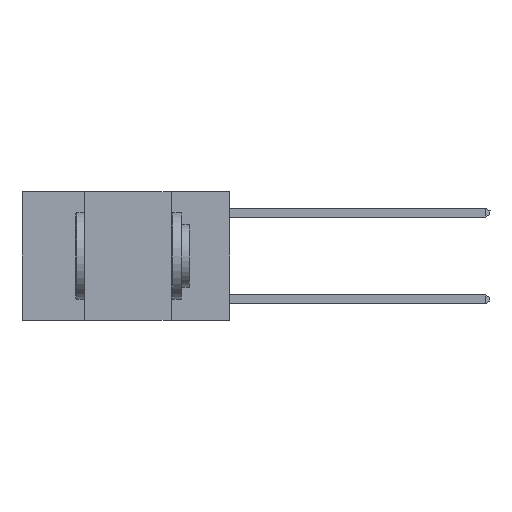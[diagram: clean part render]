
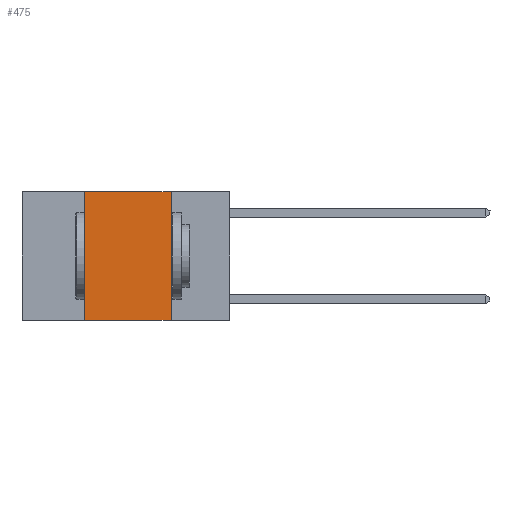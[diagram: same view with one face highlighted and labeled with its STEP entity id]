
A CAD part, left-side view. The second image highlights one B-rep face of the part: STEP entity #475.
In plain terms, the highlighted planar face has unit normal (-1, 0, 0).
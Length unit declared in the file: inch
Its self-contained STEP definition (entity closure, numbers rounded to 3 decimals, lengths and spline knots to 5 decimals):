
#241 = CARTESIAN_POINT ( 'NONE',  ( 0., 0.17, 0. ) ) ;
#475 = ADVANCED_FACE ( 'NONE', ( #7840 ), #1941, .F. ) ;
#762 = CARTESIAN_POINT ( 'NONE',  ( 0., 0.42, 0. ) ) ;
#773 = VECTOR ( 'NONE', #6024, 39.37008 ) ;
#1106 = DIRECTION ( 'NONE',  ( 0., 0., 1. ) ) ;
#1431 = CARTESIAN_POINT ( 'NONE',  ( 0., 0.6, -0.37 ) ) ;
#1667 = VERTEX_POINT ( 'NONE', #8333 ) ;
#1941 = PLANE ( 'NONE',  #8090 ) ;
#2289 = LINE ( 'NONE', #1431, #2960 ) ;
#2667 = EDGE_CURVE ( 'NONE', #1667, #3732, #8126, .T. ) ;
#2734 = DIRECTION ( 'NONE',  ( 0., 0., -1. ) ) ;
#2960 = VECTOR ( 'NONE', #9323, 39.37008 ) ;
#3459 = EDGE_CURVE ( 'NONE', #3732, #7171, #9129, .T. ) ;
#3732 = VERTEX_POINT ( 'NONE', #762 ) ;
#4145 = VECTOR ( 'NONE', #1106, 39.37008 ) ;
#4852 = DIRECTION ( 'NONE',  ( 1., 0., 0. ) ) ;
#4977 = CARTESIAN_POINT ( 'NONE',  ( 0., 0.6, 0. ) ) ;
#5039 = ORIENTED_EDGE ( 'NONE', *, *, #10826, .F. ) ;
#5040 = CARTESIAN_POINT ( 'NONE',  ( 0., 0.17, -0.37 ) ) ;
#5135 = CARTESIAN_POINT ( 'NONE',  ( 0., 0.6, 0. ) ) ;
#5699 = VERTEX_POINT ( 'NONE', #5040 ) ;
#6024 = DIRECTION ( 'NONE',  ( 0., -1., 0. ) ) ;
#7171 = VERTEX_POINT ( 'NONE', #241 ) ;
#7840 = FACE_OUTER_BOUND ( 'NONE', #10659, .T. ) ;
#8090 = AXIS2_PLACEMENT_3D ( 'NONE', #4977, #4852, #2734 ) ;
#8126 = LINE ( 'NONE', #10198, #4145 ) ;
#8333 = CARTESIAN_POINT ( 'NONE',  ( 0., 0.42, -0.37 ) ) ;
#8351 = ORIENTED_EDGE ( 'NONE', *, *, #2667, .F. ) ;
#8862 = ORIENTED_EDGE ( 'NONE', *, *, #10106, .T. ) ;
#9129 = LINE ( 'NONE', #5135, #773 ) ;
#9323 = DIRECTION ( 'NONE',  ( 0., -1., 0. ) ) ;
#9869 = ORIENTED_EDGE ( 'NONE', *, *, #3459, .F. ) ;
#10106 = EDGE_CURVE ( 'NONE', #1667, #5699, #2289, .T. ) ;
#10198 = CARTESIAN_POINT ( 'NONE',  ( 0., 0.42, 0. ) ) ;
#10638 = VECTOR ( 'NONE', #12098, 39.37008 ) ;
#10659 = EDGE_LOOP ( 'NONE', ( #5039, #9869, #8351, #8862 ) ) ;
#10826 = EDGE_CURVE ( 'NONE', #7171, #5699, #13082, .T. ) ;
#12098 = DIRECTION ( 'NONE',  ( 0., 0., -1. ) ) ;
#13021 = CARTESIAN_POINT ( 'NONE',  ( 0., 0.17, 0. ) ) ;
#13082 = LINE ( 'NONE', #13021, #10638 ) ;
